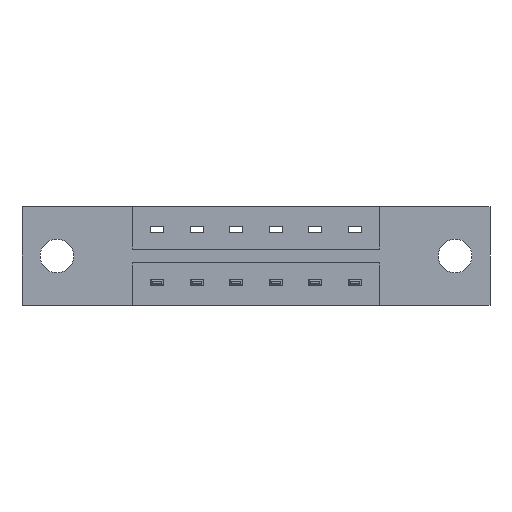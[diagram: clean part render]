
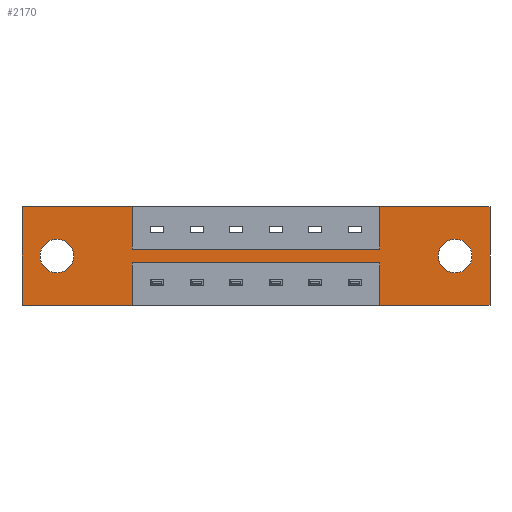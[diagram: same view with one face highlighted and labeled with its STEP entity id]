
A CAD part, front view. The second image highlights one B-rep face of the part: STEP entity #2170.
In plain terms, the highlighted planar face has unit normal (0, -1, 0).
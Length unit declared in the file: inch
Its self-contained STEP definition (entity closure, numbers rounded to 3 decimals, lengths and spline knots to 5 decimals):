
#10 = EDGE_CURVE ( 'NONE', #3413, #6560, #138, .T. ) ;
#19 = VECTOR ( 'NONE', #3212, 39.37008 ) ;
#85 = DIRECTION ( 'NONE',  ( -1., 0., 0. ) ) ;
#138 = CIRCLE ( 'NONE', #3952, 0.064 ) ;
#148 = ORIENTED_EDGE ( 'NONE', *, *, #3772, .T. ) ;
#175 = CARTESIAN_POINT ( 'NONE',  ( 1.6425, 0., -0.1235 ) ) ;
#200 = LINE ( 'NONE', #2890, #7972 ) ;
#249 = DIRECTION ( 'NONE',  ( -1., 0., 0. ) ) ;
#271 = LINE ( 'NONE', #4711, #7366 ) ;
#328 = EDGE_LOOP ( 'NONE', ( #7945, #628, #3465, #3832, #4540, #3006, #2807, #1144, #4441, #7629, #4826, #917 ) ) ;
#331 = LINE ( 'NONE', #7262, #4561 ) ;
#335 = LINE ( 'NONE', #7545, #6834 ) ;
#366 = EDGE_CURVE ( 'NONE', #3612, #6353, #331, .T. ) ;
#404 = CIRCLE ( 'NONE', #943, 0.064 ) ;
#408 = VECTOR ( 'NONE', #7772, 39.37008 ) ;
#628 = ORIENTED_EDGE ( 'NONE', *, *, #3991, .F. ) ;
#684 = CARTESIAN_POINT ( 'NONE',  ( 0.4175, 0., -0.161 ) ) ;
#778 = VECTOR ( 'NONE', #6529, 39.37008 ) ;
#883 = CARTESIAN_POINT ( 'NONE',  ( 1.775, 0., -0.375 ) ) ;
#917 = ORIENTED_EDGE ( 'NONE', *, *, #6441, .F. ) ;
#935 = VERTEX_POINT ( 'NONE', #3767 ) ;
#938 = DIRECTION ( 'NONE',  ( 1., 0., 0. ) ) ;
#943 = AXIS2_PLACEMENT_3D ( 'NONE', #6359, #6424, #1404 ) ;
#1026 = EDGE_CURVE ( 'NONE', #7247, #4683, #6717, .T. ) ;
#1028 = AXIS2_PLACEMENT_3D ( 'NONE', #4992, #3719, #6865 ) ;
#1106 = CARTESIAN_POINT ( 'NONE',  ( 1.775, 0., 0. ) ) ;
#1144 = ORIENTED_EDGE ( 'NONE', *, *, #6412, .F. ) ;
#1216 = DIRECTION ( 'NONE',  ( 0., 1., 0. ) ) ;
#1245 = CARTESIAN_POINT ( 'NONE',  ( 0.4175, 0., -0.375 ) ) ;
#1256 = EDGE_LOOP ( 'NONE', ( #7410, #148 ) ) ;
#1292 = CARTESIAN_POINT ( 'NONE',  ( 0.4175, 0., -0.214 ) ) ;
#1310 = VECTOR ( 'NONE', #4436, 39.37008 ) ;
#1399 = EDGE_LOOP ( 'NONE', ( #7314, #8026 ) ) ;
#1404 = DIRECTION ( 'NONE',  ( 0., 0., -1. ) ) ;
#1464 = CARTESIAN_POINT ( 'NONE',  ( 0.1325, 0., -0.2515 ) ) ;
#1545 = AXIS2_PLACEMENT_3D ( 'NONE', #3307, #4625, #3967 ) ;
#1781 = CARTESIAN_POINT ( 'NONE',  ( 1.6425, 0., -0.1875 ) ) ;
#1800 = VERTEX_POINT ( 'NONE', #2228 ) ;
#1825 = EDGE_CURVE ( 'NONE', #8161, #935, #6601, .T. ) ;
#1970 = VERTEX_POINT ( 'NONE', #4398 ) ;
#2170 = ADVANCED_FACE ( 'NONE', ( #3470, #2771, #4659 ), #5810, .T. ) ;
#2228 = CARTESIAN_POINT ( 'NONE',  ( 1.3575, 0., 0. ) ) ;
#2460 = DIRECTION ( 'NONE',  ( 1., 0., 0. ) ) ;
#2482 = VERTEX_POINT ( 'NONE', #5308 ) ;
#2592 = VERTEX_POINT ( 'NONE', #684 ) ;
#2771 = FACE_BOUND ( 'NONE', #1256, .T. ) ;
#2807 = ORIENTED_EDGE ( 'NONE', *, *, #4085, .F. ) ;
#2832 = VECTOR ( 'NONE', #249, 39.37008 ) ;
#2890 = CARTESIAN_POINT ( 'NONE',  ( 1.3575, 0., -0.161 ) ) ;
#3006 = ORIENTED_EDGE ( 'NONE', *, *, #4852, .F. ) ;
#3087 = VECTOR ( 'NONE', #4316, 39.37008 ) ;
#3199 = CARTESIAN_POINT ( 'NONE',  ( 0.4175, 0., -0.214 ) ) ;
#3212 = DIRECTION ( 'NONE',  ( 0., 0., -1. ) ) ;
#3267 = VERTEX_POINT ( 'NONE', #175 ) ;
#3307 = CARTESIAN_POINT ( 'NONE',  ( 0., 0., -0.375 ) ) ;
#3413 = VERTEX_POINT ( 'NONE', #5944 ) ;
#3465 = ORIENTED_EDGE ( 'NONE', *, *, #1026, .F. ) ;
#3470 = FACE_BOUND ( 'NONE', #1399, .T. ) ;
#3612 = VERTEX_POINT ( 'NONE', #4908 ) ;
#3661 = DIRECTION ( 'NONE',  ( 0., 0., -1. ) ) ;
#3719 = DIRECTION ( 'NONE',  ( 0., 1., 0. ) ) ;
#3767 = CARTESIAN_POINT ( 'NONE',  ( 0., 0., 0. ) ) ;
#3772 = EDGE_CURVE ( 'NONE', #6560, #3413, #4226, .T. ) ;
#3821 = LINE ( 'NONE', #5876, #2832 ) ;
#3832 = ORIENTED_EDGE ( 'NONE', *, *, #5160, .F. ) ;
#3840 = CARTESIAN_POINT ( 'NONE',  ( 1.3575, 0., -0.161 ) ) ;
#3952 = AXIS2_PLACEMENT_3D ( 'NONE', #7117, #5446, #6511 ) ;
#3956 = CARTESIAN_POINT ( 'NONE',  ( 1.775, 0., 0. ) ) ;
#3967 = DIRECTION ( 'NONE',  ( 0., 0., -1. ) ) ;
#3991 = EDGE_CURVE ( 'NONE', #4683, #3612, #3821, .T. ) ;
#4085 = EDGE_CURVE ( 'NONE', #5589, #2592, #4120, .T. ) ;
#4120 = LINE ( 'NONE', #7750, #778 ) ;
#4144 = DIRECTION ( 'NONE',  ( 0., 0., 1. ) ) ;
#4226 = CIRCLE ( 'NONE', #1028, 0.064 ) ;
#4316 = DIRECTION ( 'NONE',  ( -1., 0., 0. ) ) ;
#4398 = CARTESIAN_POINT ( 'NONE',  ( 0.4175, 0., -0.214 ) ) ;
#4436 = DIRECTION ( 'NONE',  ( 1., 0., 0. ) ) ;
#4441 = ORIENTED_EDGE ( 'NONE', *, *, #1825, .F. ) ;
#4540 = ORIENTED_EDGE ( 'NONE', *, *, #7894, .F. ) ;
#4557 = LINE ( 'NONE', #1292, #19 ) ;
#4561 = VECTOR ( 'NONE', #4144, 39.37008 ) ;
#4625 = DIRECTION ( 'NONE',  ( 0., -1., 0. ) ) ;
#4659 = FACE_OUTER_BOUND ( 'NONE', #328, .T. ) ;
#4683 = VERTEX_POINT ( 'NONE', #883 ) ;
#4711 = CARTESIAN_POINT ( 'NONE',  ( 0.4175, 0., -0.161 ) ) ;
#4826 = ORIENTED_EDGE ( 'NONE', *, *, #7054, .F. ) ;
#4852 = EDGE_CURVE ( 'NONE', #2592, #5337, #271, .T. ) ;
#4908 = CARTESIAN_POINT ( 'NONE',  ( 1.3575, 0., -0.375 ) ) ;
#4951 = EDGE_CURVE ( 'NONE', #7385, #8161, #7228, .T. ) ;
#4992 = CARTESIAN_POINT ( 'NONE',  ( 0.1325, 0., -0.1875 ) ) ;
#5057 = CARTESIAN_POINT ( 'NONE',  ( 0., 0., 0. ) ) ;
#5154 = VECTOR ( 'NONE', #85, 39.37008 ) ;
#5160 = EDGE_CURVE ( 'NONE', #1800, #7247, #335, .T. ) ;
#5308 = CARTESIAN_POINT ( 'NONE',  ( 1.6425, 0., -0.2515 ) ) ;
#5337 = VERTEX_POINT ( 'NONE', #3840 ) ;
#5429 = VECTOR ( 'NONE', #5456, 39.37008 ) ;
#5446 = DIRECTION ( 'NONE',  ( 0., 1., 0. ) ) ;
#5456 = DIRECTION ( 'NONE',  ( 0., 0., 1. ) ) ;
#5589 = VERTEX_POINT ( 'NONE', #7370 ) ;
#5728 = CIRCLE ( 'NONE', #6746, 0.064 ) ;
#5738 = LINE ( 'NONE', #3199, #5154 ) ;
#5810 = PLANE ( 'NONE',  #1545 ) ;
#5876 = CARTESIAN_POINT ( 'NONE',  ( 0., 0., -0.375 ) ) ;
#5944 = CARTESIAN_POINT ( 'NONE',  ( 0.1325, 0., -0.1235 ) ) ;
#6296 = CARTESIAN_POINT ( 'NONE',  ( 0., 0., -0.375 ) ) ;
#6353 = VERTEX_POINT ( 'NONE', #8063 ) ;
#6359 = CARTESIAN_POINT ( 'NONE',  ( 1.6425, 0., -0.1875 ) ) ;
#6412 = EDGE_CURVE ( 'NONE', #935, #5589, #8095, .T. ) ;
#6424 = DIRECTION ( 'NONE',  ( 0., 1., 0. ) ) ;
#6441 = EDGE_CURVE ( 'NONE', #6353, #1970, #5738, .T. ) ;
#6511 = DIRECTION ( 'NONE',  ( 0., 0., 1. ) ) ;
#6529 = DIRECTION ( 'NONE',  ( 0., 0., -1. ) ) ;
#6560 = VERTEX_POINT ( 'NONE', #1464 ) ;
#6601 = LINE ( 'NONE', #7830, #5429 ) ;
#6689 = DIRECTION ( 'NONE',  ( 0., 0., 1. ) ) ;
#6717 = LINE ( 'NONE', #3956, #408 ) ;
#6723 = CARTESIAN_POINT ( 'NONE',  ( 0., 0., -0.375 ) ) ;
#6746 = AXIS2_PLACEMENT_3D ( 'NONE', #1781, #1216, #3661 ) ;
#6834 = VECTOR ( 'NONE', #2460, 39.37008 ) ;
#6865 = DIRECTION ( 'NONE',  ( 0., 0., 1. ) ) ;
#6956 = EDGE_CURVE ( 'NONE', #3267, #2482, #5728, .T. ) ;
#7054 = EDGE_CURVE ( 'NONE', #1970, #7385, #4557, .T. ) ;
#7117 = CARTESIAN_POINT ( 'NONE',  ( 0.1325, 0., -0.1875 ) ) ;
#7141 = EDGE_CURVE ( 'NONE', #2482, #3267, #404, .T. ) ;
#7228 = LINE ( 'NONE', #6723, #3087 ) ;
#7247 = VERTEX_POINT ( 'NONE', #1106 ) ;
#7262 = CARTESIAN_POINT ( 'NONE',  ( 1.3575, 0., -0.214 ) ) ;
#7314 = ORIENTED_EDGE ( 'NONE', *, *, #6956, .T. ) ;
#7366 = VECTOR ( 'NONE', #938, 39.37008 ) ;
#7370 = CARTESIAN_POINT ( 'NONE',  ( 0.4175, 0., 0. ) ) ;
#7385 = VERTEX_POINT ( 'NONE', #1245 ) ;
#7410 = ORIENTED_EDGE ( 'NONE', *, *, #10, .T. ) ;
#7545 = CARTESIAN_POINT ( 'NONE',  ( 0., 0., 0. ) ) ;
#7629 = ORIENTED_EDGE ( 'NONE', *, *, #4951, .F. ) ;
#7750 = CARTESIAN_POINT ( 'NONE',  ( 0.4175, 0., -0.161 ) ) ;
#7772 = DIRECTION ( 'NONE',  ( 0., 0., -1. ) ) ;
#7830 = CARTESIAN_POINT ( 'NONE',  ( 0., 0., 0. ) ) ;
#7894 = EDGE_CURVE ( 'NONE', #5337, #1800, #200, .T. ) ;
#7945 = ORIENTED_EDGE ( 'NONE', *, *, #366, .F. ) ;
#7972 = VECTOR ( 'NONE', #6689, 39.37008 ) ;
#8026 = ORIENTED_EDGE ( 'NONE', *, *, #7141, .T. ) ;
#8063 = CARTESIAN_POINT ( 'NONE',  ( 1.3575, 0., -0.214 ) ) ;
#8095 = LINE ( 'NONE', #5057, #1310 ) ;
#8161 = VERTEX_POINT ( 'NONE', #6296 ) ;
